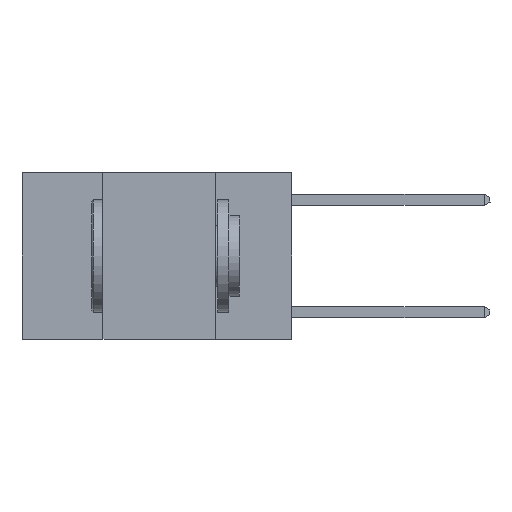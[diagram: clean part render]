
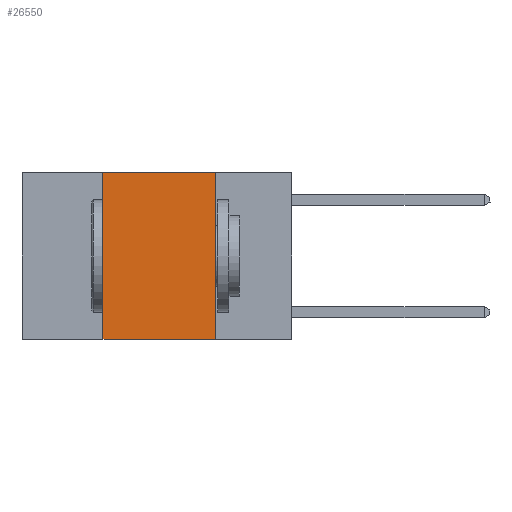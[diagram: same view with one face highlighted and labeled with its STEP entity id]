
A CAD part, left-side view. The second image highlights one B-rep face of the part: STEP entity #26550.
In plain terms, the highlighted planar face has unit normal (-1, 0, 0).
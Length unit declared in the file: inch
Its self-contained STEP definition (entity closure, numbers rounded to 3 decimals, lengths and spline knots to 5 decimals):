
#587 = VECTOR ( 'NONE', #10565, 39.37008 ) ;
#1068 = CARTESIAN_POINT ( 'NONE',  ( 0., 0.17, -0.37 ) ) ;
#1586 = CARTESIAN_POINT ( 'NONE',  ( 0., 0.6, -0.37 ) ) ;
#3316 = VECTOR ( 'NONE', #9216, 39.37008 ) ;
#4712 = EDGE_CURVE ( 'NONE', #22739, #16031, #23277, .T. ) ;
#5487 = VECTOR ( 'NONE', #24411, 39.37008 ) ;
#5537 = PLANE ( 'NONE',  #23336 ) ;
#6197 = EDGE_CURVE ( 'NONE', #23771, #25347, #15244, .T. ) ;
#6505 = CARTESIAN_POINT ( 'NONE',  ( 0., 0.42, 0. ) ) ;
#6783 = EDGE_LOOP ( 'NONE', ( #24804, #8483, #26174, #9914 ) ) ;
#6926 = CARTESIAN_POINT ( 'NONE',  ( 0., 0.17, 0. ) ) ;
#7815 = CARTESIAN_POINT ( 'NONE',  ( 0., 0.6, 0. ) ) ;
#8483 = ORIENTED_EDGE ( 'NONE', *, *, #13948, .F. ) ;
#9216 = DIRECTION ( 'NONE',  ( 0., 0., -1. ) ) ;
#9832 = FACE_OUTER_BOUND ( 'NONE', #6783, .T. ) ;
#9914 = ORIENTED_EDGE ( 'NONE', *, *, #10771, .T. ) ;
#10098 = DIRECTION ( 'NONE',  ( 1., 0., 0. ) ) ;
#10245 = CARTESIAN_POINT ( 'NONE',  ( 0., 0.6, 0. ) ) ;
#10565 = DIRECTION ( 'NONE',  ( 0., -1., 0. ) ) ;
#10771 = EDGE_CURVE ( 'NONE', #22739, #25347, #18457, .T. ) ;
#11070 = LINE ( 'NONE', #10245, #22175 ) ;
#13572 = CARTESIAN_POINT ( 'NONE',  ( 0., 0.17, 0. ) ) ;
#13948 = EDGE_CURVE ( 'NONE', #16031, #23771, #11070, .T. ) ;
#15244 = LINE ( 'NONE', #6926, #3316 ) ;
#16031 = VERTEX_POINT ( 'NONE', #21307 ) ;
#18457 = LINE ( 'NONE', #1586, #587 ) ;
#21307 = CARTESIAN_POINT ( 'NONE',  ( 0., 0.42, 0. ) ) ;
#22175 = VECTOR ( 'NONE', #27875, 39.37008 ) ;
#22739 = VERTEX_POINT ( 'NONE', #27808 ) ;
#23277 = LINE ( 'NONE', #6505, #5487 ) ;
#23336 = AXIS2_PLACEMENT_3D ( 'NONE', #7815, #10098, #25589 ) ;
#23771 = VERTEX_POINT ( 'NONE', #13572 ) ;
#24411 = DIRECTION ( 'NONE',  ( 0., 0., 1. ) ) ;
#24804 = ORIENTED_EDGE ( 'NONE', *, *, #6197, .F. ) ;
#25347 = VERTEX_POINT ( 'NONE', #1068 ) ;
#25589 = DIRECTION ( 'NONE',  ( 0., 0., -1. ) ) ;
#26174 = ORIENTED_EDGE ( 'NONE', *, *, #4712, .F. ) ;
#26550 = ADVANCED_FACE ( 'NONE', ( #9832 ), #5537, .F. ) ;
#27808 = CARTESIAN_POINT ( 'NONE',  ( 0., 0.42, -0.37 ) ) ;
#27875 = DIRECTION ( 'NONE',  ( 0., -1., 0. ) ) ;
